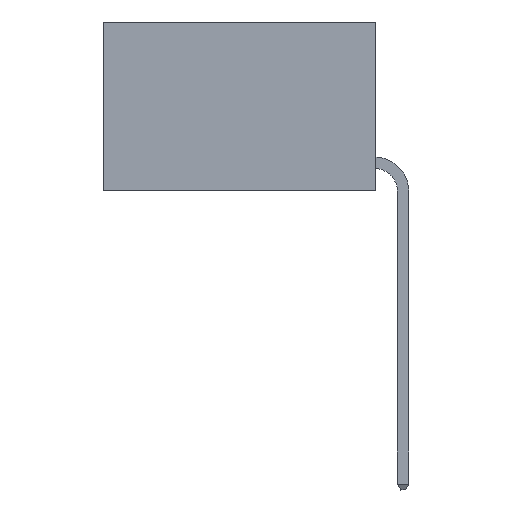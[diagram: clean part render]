
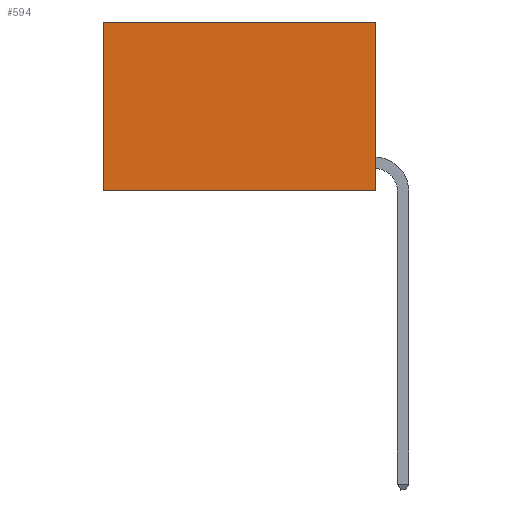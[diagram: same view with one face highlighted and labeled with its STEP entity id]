
A CAD part, left-side view. The second image highlights one B-rep face of the part: STEP entity #594.
In plain terms, the highlighted planar face has unit normal (-1, 0, 0).
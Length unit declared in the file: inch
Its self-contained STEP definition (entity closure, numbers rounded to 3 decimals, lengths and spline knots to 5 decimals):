
#469 = VECTOR ( 'NONE', #2250, 39.37008 ) ;
#475 = ORIENTED_EDGE ( 'NONE', *, *, #9493, .F. ) ;
#578 = CARTESIAN_POINT ( 'NONE',  ( 0.2625, 0.6, 0. ) ) ;
#594 = ADVANCED_FACE ( 'NONE', ( #5482 ), #7469, .F. ) ;
#962 = CARTESIAN_POINT ( 'NONE',  ( 0.2625, 0., 0. ) ) ;
#1099 = EDGE_LOOP ( 'NONE', ( #6235, #3762, #475, #9392 ) ) ;
#1165 = CARTESIAN_POINT ( 'NONE',  ( 0.2625, 0.6, -0.37 ) ) ;
#1375 = DIRECTION ( 'NONE',  ( 0., 0., -1. ) ) ;
#1631 = VECTOR ( 'NONE', #6233, 39.37008 ) ;
#1660 = EDGE_CURVE ( 'NONE', #6479, #7921, #4201, .T. ) ;
#2247 = EDGE_CURVE ( 'NONE', #9023, #5723, #4400, .T. ) ;
#2250 = DIRECTION ( 'NONE',  ( 0., 1., 0. ) ) ;
#2770 = LINE ( 'NONE', #962, #1631 ) ;
#3762 = ORIENTED_EDGE ( 'NONE', *, *, #2247, .F. ) ;
#4155 = EDGE_CURVE ( 'NONE', #7921, #5723, #7451, .T. ) ;
#4201 = LINE ( 'NONE', #10103, #469 ) ;
#4400 = LINE ( 'NONE', #8655, #8008 ) ;
#4464 = VECTOR ( 'NONE', #4946, 39.37008 ) ;
#4946 = DIRECTION ( 'NONE',  ( 0., 0., -1. ) ) ;
#5482 = FACE_OUTER_BOUND ( 'NONE', #1099, .T. ) ;
#5723 = VERTEX_POINT ( 'NONE', #1165 ) ;
#6233 = DIRECTION ( 'NONE',  ( 0., 0., -1. ) ) ;
#6235 = ORIENTED_EDGE ( 'NONE', *, *, #4155, .T. ) ;
#6467 = CARTESIAN_POINT ( 'NONE',  ( 0.2625, 0., 0. ) ) ;
#6479 = VERTEX_POINT ( 'NONE', #6467 ) ;
#6946 = CARTESIAN_POINT ( 'NONE',  ( 0.2625, 0., -0.37 ) ) ;
#7451 = LINE ( 'NONE', #578, #4464 ) ;
#7469 = PLANE ( 'NONE',  #8639 ) ;
#7781 = DIRECTION ( 'NONE',  ( 0., 1., 0. ) ) ;
#7921 = VERTEX_POINT ( 'NONE', #10980 ) ;
#8008 = VECTOR ( 'NONE', #7781, 39.37008 ) ;
#8113 = CARTESIAN_POINT ( 'NONE',  ( 0.2625, 0., 0. ) ) ;
#8639 = AXIS2_PLACEMENT_3D ( 'NONE', #8113, #10018, #1375 ) ;
#8655 = CARTESIAN_POINT ( 'NONE',  ( 0.2625, 0., -0.37 ) ) ;
#9023 = VERTEX_POINT ( 'NONE', #6946 ) ;
#9392 = ORIENTED_EDGE ( 'NONE', *, *, #1660, .T. ) ;
#9493 = EDGE_CURVE ( 'NONE', #6479, #9023, #2770, .T. ) ;
#10018 = DIRECTION ( 'NONE',  ( 1., 0., 0. ) ) ;
#10103 = CARTESIAN_POINT ( 'NONE',  ( 0.2625, 0., 0. ) ) ;
#10980 = CARTESIAN_POINT ( 'NONE',  ( 0.2625, 0.6, 0. ) ) ;
